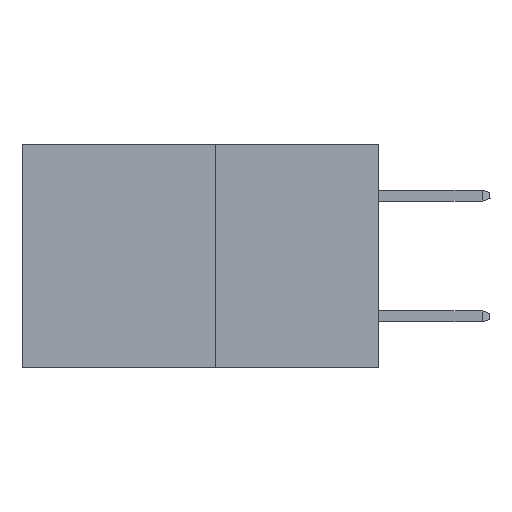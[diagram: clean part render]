
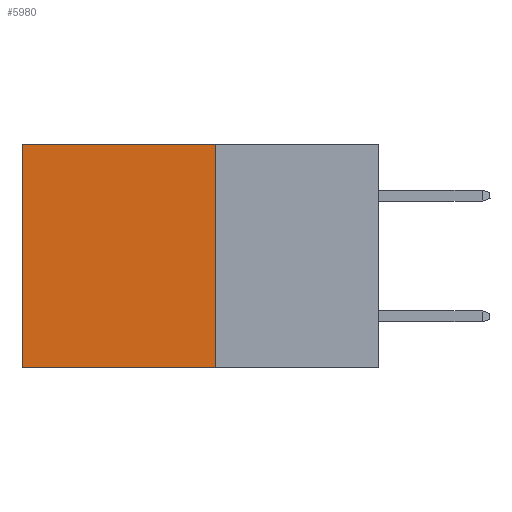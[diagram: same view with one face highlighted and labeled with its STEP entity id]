
A CAD part, left-side view. The second image highlights one B-rep face of the part: STEP entity #5980.
In plain terms, the highlighted planar face has unit normal (-1, 0, 0).
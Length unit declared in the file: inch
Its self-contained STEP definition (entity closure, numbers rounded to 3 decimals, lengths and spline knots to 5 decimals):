
#1500 = CARTESIAN_POINT ( 'NONE',  ( 0.277, 0.59, -0.37 ) ) ;
#2610 = EDGE_CURVE ( 'NONE', #11893, #23452, #21764, .T. ) ;
#3235 = EDGE_CURVE ( 'NONE', #25992, #11893, #22932, .T. ) ;
#3471 = DIRECTION ( 'NONE',  ( 0., 1., 0. ) ) ;
#3707 = ORIENTED_EDGE ( 'NONE', *, *, #3235, .F. ) ;
#4654 = VECTOR ( 'NONE', #3471, 39.37008 ) ;
#5980 = ADVANCED_FACE ( 'NONE', ( #13198 ), #18662, .F. ) ;
#6326 = LINE ( 'NONE', #21997, #4654 ) ;
#6366 = EDGE_CURVE ( 'NONE', #33390, #23452, #21053, .T. ) ;
#6919 = VECTOR ( 'NONE', #8282, 39.37008 ) ;
#8282 = DIRECTION ( 'NONE',  ( 0., 0., -1. ) ) ;
#11893 = VERTEX_POINT ( 'NONE', #16498 ) ;
#12092 = CARTESIAN_POINT ( 'NONE',  ( 0.277, 0.59, -0.37 ) ) ;
#12696 = CARTESIAN_POINT ( 'NONE',  ( 0.277, 0.27, -0.37 ) ) ;
#13198 = FACE_OUTER_BOUND ( 'NONE', #16556, .T. ) ;
#13500 = CARTESIAN_POINT ( 'NONE',  ( 0.277, 0.27, -0.37 ) ) ;
#15120 = VECTOR ( 'NONE', #17071, 39.37008 ) ;
#16020 = ORIENTED_EDGE ( 'NONE', *, *, #6366, .T. ) ;
#16498 = CARTESIAN_POINT ( 'NONE',  ( 0.277, 0.27, -0.37 ) ) ;
#16556 = EDGE_LOOP ( 'NONE', ( #16020, #23934, #3707, #31577 ) ) ;
#17071 = DIRECTION ( 'NONE',  ( 0., 0., -1. ) ) ;
#17380 = DIRECTION ( 'NONE',  ( 0., 0., -1. ) ) ;
#18662 = PLANE ( 'NONE',  #33839 ) ;
#18798 = CARTESIAN_POINT ( 'NONE',  ( 0.277, 0.27, -0.37 ) ) ;
#21053 = LINE ( 'NONE', #12092, #6919 ) ;
#21764 = LINE ( 'NONE', #12696, #27832 ) ;
#21997 = CARTESIAN_POINT ( 'NONE',  ( 0.277, 0.27, 0. ) ) ;
#22401 = CARTESIAN_POINT ( 'NONE',  ( 0.277, 0.59, 0. ) ) ;
#22932 = LINE ( 'NONE', #13500, #15120 ) ;
#23452 = VERTEX_POINT ( 'NONE', #1500 ) ;
#23934 = ORIENTED_EDGE ( 'NONE', *, *, #2610, .F. ) ;
#25992 = VERTEX_POINT ( 'NONE', #31434 ) ;
#27832 = VECTOR ( 'NONE', #33252, 39.37008 ) ;
#29362 = DIRECTION ( 'NONE',  ( 1., 0., 0. ) ) ;
#30016 = EDGE_CURVE ( 'NONE', #25992, #33390, #6326, .T. ) ;
#31434 = CARTESIAN_POINT ( 'NONE',  ( 0.277, 0.27, 0. ) ) ;
#31577 = ORIENTED_EDGE ( 'NONE', *, *, #30016, .T. ) ;
#33252 = DIRECTION ( 'NONE',  ( 0., 1., 0. ) ) ;
#33390 = VERTEX_POINT ( 'NONE', #22401 ) ;
#33839 = AXIS2_PLACEMENT_3D ( 'NONE', #18798, #29362, #17380 ) ;
